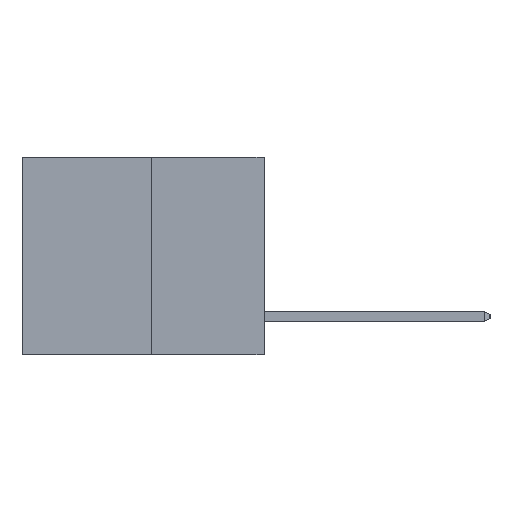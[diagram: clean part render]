
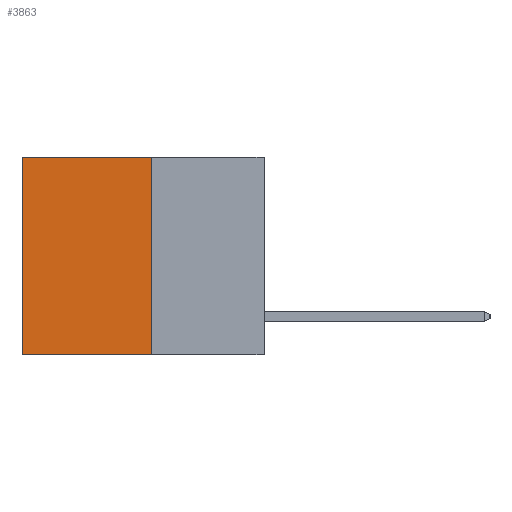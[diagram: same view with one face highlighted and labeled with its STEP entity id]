
A CAD part, left-side view. The second image highlights one B-rep face of the part: STEP entity #3863.
In plain terms, the highlighted planar face has unit normal (-1, 0, 0).
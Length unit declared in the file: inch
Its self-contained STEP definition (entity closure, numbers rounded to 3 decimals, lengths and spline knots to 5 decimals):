
#1663 = CARTESIAN_POINT ( 'NONE',  ( 0.3165, 0.6, 0. ) ) ;
#1945 = CARTESIAN_POINT ( 'NONE',  ( 0.3165, 0.28, -0.49 ) ) ;
#2339 = LINE ( 'NONE', #2762, #14102 ) ;
#2762 = CARTESIAN_POINT ( 'NONE',  ( 0.3165, 0.28, -0.49 ) ) ;
#2792 = ORIENTED_EDGE ( 'NONE', *, *, #16837, .T. ) ;
#3863 = ADVANCED_FACE ( 'NONE', ( #16934 ), #9669, .F. ) ;
#4592 = DIRECTION ( 'NONE',  ( 0., 0., -1. ) ) ;
#4828 = DIRECTION ( 'NONE',  ( 0., 1., 0. ) ) ;
#5404 = LINE ( 'NONE', #9358, #5901 ) ;
#5901 = VECTOR ( 'NONE', #4828, 39.37008 ) ;
#7752 = VECTOR ( 'NONE', #4592, 39.37008 ) ;
#8023 = DIRECTION ( 'NONE',  ( 0., 0., -1. ) ) ;
#8041 = EDGE_CURVE ( 'NONE', #12127, #15812, #2339, .T. ) ;
#8214 = LINE ( 'NONE', #14550, #7752 ) ;
#9358 = CARTESIAN_POINT ( 'NONE',  ( 0.3165, 0.28, 0. ) ) ;
#9382 = EDGE_LOOP ( 'NONE', ( #17765, #9571, #15597, #2792 ) ) ;
#9543 = AXIS2_PLACEMENT_3D ( 'NONE', #1945, #14116, #8023 ) ;
#9571 = ORIENTED_EDGE ( 'NONE', *, *, #19336, .F. ) ;
#9669 = PLANE ( 'NONE',  #9543 ) ;
#11621 = EDGE_CURVE ( 'NONE', #18946, #18728, #8214, .T. ) ;
#11716 = CARTESIAN_POINT ( 'NONE',  ( 0.3165, 0.28, 0. ) ) ;
#12010 = CARTESIAN_POINT ( 'NONE',  ( 0.3165, 0.28, -0.49 ) ) ;
#12038 = VECTOR ( 'NONE', #16649, 39.37008 ) ;
#12043 = DIRECTION ( 'NONE',  ( 0., 0., -1. ) ) ;
#12127 = VERTEX_POINT ( 'NONE', #11716 ) ;
#14102 = VECTOR ( 'NONE', #12043, 39.37008 ) ;
#14116 = DIRECTION ( 'NONE',  ( 1., 0., 0. ) ) ;
#14550 = CARTESIAN_POINT ( 'NONE',  ( 0.3165, 0.6, -0.49 ) ) ;
#15597 = ORIENTED_EDGE ( 'NONE', *, *, #8041, .F. ) ;
#15812 = VERTEX_POINT ( 'NONE', #17737 ) ;
#16649 = DIRECTION ( 'NONE',  ( 0., 1., 0. ) ) ;
#16837 = EDGE_CURVE ( 'NONE', #12127, #18946, #5404, .T. ) ;
#16934 = FACE_OUTER_BOUND ( 'NONE', #9382, .T. ) ;
#17737 = CARTESIAN_POINT ( 'NONE',  ( 0.3165, 0.28, -0.49 ) ) ;
#17765 = ORIENTED_EDGE ( 'NONE', *, *, #11621, .T. ) ;
#18728 = VERTEX_POINT ( 'NONE', #19763 ) ;
#18946 = VERTEX_POINT ( 'NONE', #1663 ) ;
#19336 = EDGE_CURVE ( 'NONE', #15812, #18728, #19728, .T. ) ;
#19728 = LINE ( 'NONE', #12010, #12038 ) ;
#19763 = CARTESIAN_POINT ( 'NONE',  ( 0.3165, 0.6, -0.49 ) ) ;
